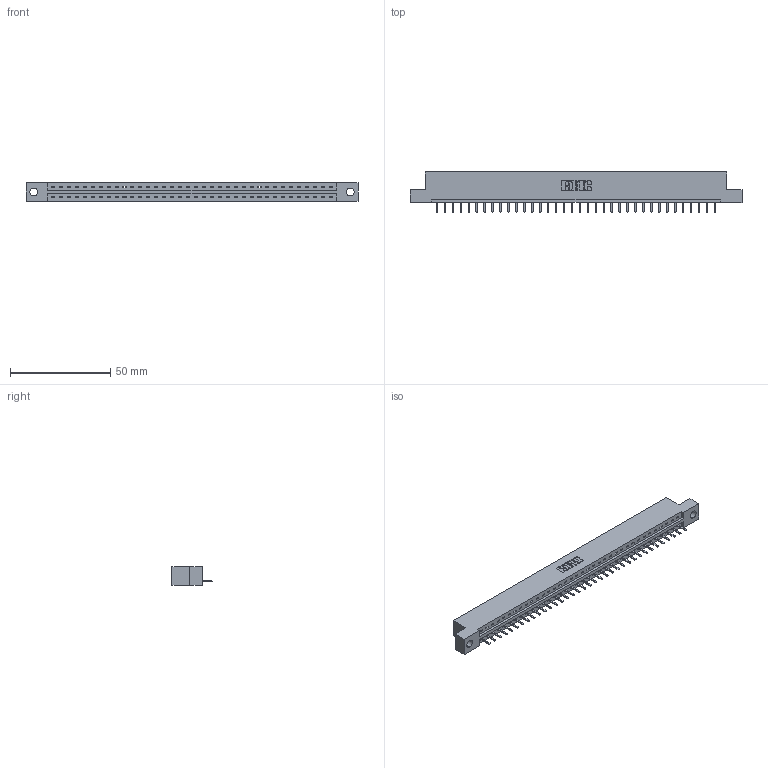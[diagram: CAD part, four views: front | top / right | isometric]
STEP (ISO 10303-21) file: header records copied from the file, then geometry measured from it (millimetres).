
FILE_DESCRIPTION (( 'STEP AP203' ), '1' );
FILE_NAME ('387-036-520-104.STEP', '2018-09-18T23:05:40', ( '' ), ( '' ), 'SwSTEP 2.0', 'SolidWorks 2016', '' );
FILE_SCHEMA (( 'CONFIG_CONTROL_DESIGN' ));
Length unit declared in the file: inch
Products named in the file (3): 337 Part_Flush Mounting Lugs - 0.156 Dia-TH; 345-292-001_345-293-120; 387-036-520-104
Assembly tree (37 placements, depth 2):
  387-036-520-104
    337 Part_Flush Mounting Lugs - 0.156 Dia-TH
    345-292-001_345-293-120  x36
Bounding box: 165.66 x 20.02 x 9.4 mm (x, y, z)
Volume: 16951 mm3; surface area: 16905.5 mm2
Topology: 37 solids, 37 shells, 2490 faces, 7367 edges, 4814 vertices
Faces by surface type: plane 1798, cylinder 692
Entity records: 27653 total; most frequent: CARTESIAN_POINT 4834, ORIENTED_EDGE 4794, DIRECTION 4069, EDGE_CURVE 2397, LINE 2265, VECTOR 2265, VERTEX_POINT 1594, AXIS2_PLACEMENT_3D 902
